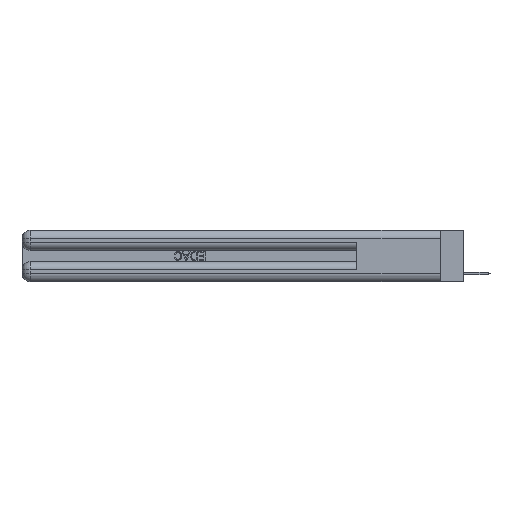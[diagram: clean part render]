
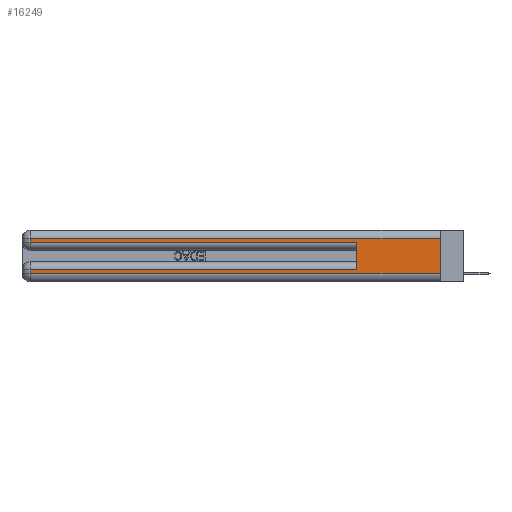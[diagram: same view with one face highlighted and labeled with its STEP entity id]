
A CAD part, left-side view. The second image highlights one B-rep face of the part: STEP entity #16249.
In plain terms, the highlighted planar face has unit normal (-1, 0, 0).
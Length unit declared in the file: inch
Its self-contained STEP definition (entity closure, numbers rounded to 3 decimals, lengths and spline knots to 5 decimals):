
#4 = ORIENTED_EDGE ( 'NONE', *, *, #17912, .T. ) ;
#371 = VERTEX_POINT ( 'NONE', #3108 ) ;
#781 = CARTESIAN_POINT ( 'NONE',  ( 0., 2.94, 0.06 ) ) ;
#1278 = CARTESIAN_POINT ( 'NONE',  ( 0., 2.94, 0.37 ) ) ;
#1391 = ORIENTED_EDGE ( 'NONE', *, *, #12706, .T. ) ;
#1417 = DIRECTION ( 'NONE',  ( 0., 0., -1. ) ) ;
#2069 = LINE ( 'NONE', #6868, #9115 ) ;
#2328 = ORIENTED_EDGE ( 'NONE', *, *, #8604, .T. ) ;
#2939 = VERTEX_POINT ( 'NONE', #16931 ) ;
#3108 = CARTESIAN_POINT ( 'NONE',  ( 0., 0.6, 0.085 ) ) ;
#4401 = EDGE_CURVE ( 'NONE', #371, #8833, #24766, .T. ) ;
#4469 = CARTESIAN_POINT ( 'NONE',  ( 0., 0., 0.06 ) ) ;
#4558 = CARTESIAN_POINT ( 'NONE',  ( 0., 0., 0.085 ) ) ;
#5405 = LINE ( 'NONE', #18814, #28959 ) ;
#5949 = CARTESIAN_POINT ( 'NONE',  ( 0., 0., 0.31 ) ) ;
#5952 = EDGE_CURVE ( 'NONE', #21578, #17408, #10750, .T. ) ;
#6176 = FACE_OUTER_BOUND ( 'NONE', #17130, .T. ) ;
#6374 = AXIS2_PLACEMENT_3D ( 'NONE', #22538, #29433, #15670 ) ;
#6868 = CARTESIAN_POINT ( 'NONE',  ( 0., 2.94, 0.37 ) ) ;
#6993 = VERTEX_POINT ( 'NONE', #17894 ) ;
#8342 = DIRECTION ( 'NONE',  ( 0., 0., 1. ) ) ;
#8559 = VECTOR ( 'NONE', #19491, 39.37008 ) ;
#8604 = EDGE_CURVE ( 'NONE', #27648, #17408, #28616, .T. ) ;
#8833 = VERTEX_POINT ( 'NONE', #12142 ) ;
#9115 = VECTOR ( 'NONE', #11151, 39.37008 ) ;
#9828 = ORIENTED_EDGE ( 'NONE', *, *, #4401, .F. ) ;
#10750 = LINE ( 'NONE', #19885, #12065 ) ;
#10819 = DIRECTION ( 'NONE',  ( 0., -1., 0. ) ) ;
#11151 = DIRECTION ( 'NONE',  ( 0., 0., -1. ) ) ;
#11373 = LINE ( 'NONE', #4558, #29319 ) ;
#11466 = VECTOR ( 'NONE', #10819, 39.37008 ) ;
#12065 = VECTOR ( 'NONE', #14960, 39.37008 ) ;
#12142 = CARTESIAN_POINT ( 'NONE',  ( 0., 0.6, 0.285 ) ) ;
#12706 = EDGE_CURVE ( 'NONE', #2939, #8833, #5405, .T. ) ;
#12940 = ORIENTED_EDGE ( 'NONE', *, *, #5952, .F. ) ;
#13879 = CARTESIAN_POINT ( 'NONE',  ( 0., 0., 0.31 ) ) ;
#14464 = DIRECTION ( 'NONE',  ( 0., -1., 0. ) ) ;
#14960 = DIRECTION ( 'NONE',  ( 0., 0., -1. ) ) ;
#15670 = DIRECTION ( 'NONE',  ( 0., 0., -1. ) ) ;
#16249 = ADVANCED_FACE ( 'NONE', ( #6176 ), #24799, .F. ) ;
#16931 = CARTESIAN_POINT ( 'NONE',  ( 0., 2.94, 0.285 ) ) ;
#17130 = EDGE_LOOP ( 'NONE', ( #12940, #20433, #24268, #1391, #9828, #4, #25158, #2328 ) ) ;
#17408 = VERTEX_POINT ( 'NONE', #4469 ) ;
#17894 = CARTESIAN_POINT ( 'NONE',  ( 0., 2.94, 0.085 ) ) ;
#17912 = EDGE_CURVE ( 'NONE', #371, #6993, #11373, .T. ) ;
#18814 = CARTESIAN_POINT ( 'NONE',  ( 0., 0., 0.285 ) ) ;
#19491 = DIRECTION ( 'NONE',  ( 0., 1., 0. ) ) ;
#19885 = CARTESIAN_POINT ( 'NONE',  ( 0., 0., 0.37 ) ) ;
#19943 = LINE ( 'NONE', #5949, #8559 ) ;
#19953 = CARTESIAN_POINT ( 'NONE',  ( 0., 2.94, 0.31 ) ) ;
#20433 = ORIENTED_EDGE ( 'NONE', *, *, #27905, .T. ) ;
#21557 = EDGE_CURVE ( 'NONE', #6993, #27648, #21728, .T. ) ;
#21578 = VERTEX_POINT ( 'NONE', #13879 ) ;
#21728 = LINE ( 'NONE', #1278, #27260 ) ;
#21902 = CARTESIAN_POINT ( 'NONE',  ( 0., 0.6, 0.145 ) ) ;
#22538 = CARTESIAN_POINT ( 'NONE',  ( 0., 0., 0.37 ) ) ;
#22578 = EDGE_CURVE ( 'NONE', #23117, #2939, #2069, .T. ) ;
#23117 = VERTEX_POINT ( 'NONE', #19953 ) ;
#24268 = ORIENTED_EDGE ( 'NONE', *, *, #22578, .T. ) ;
#24766 = LINE ( 'NONE', #21902, #27703 ) ;
#24799 = PLANE ( 'NONE',  #6374 ) ;
#25158 = ORIENTED_EDGE ( 'NONE', *, *, #21557, .T. ) ;
#26679 = CARTESIAN_POINT ( 'NONE',  ( 0., 0., 0.06 ) ) ;
#27260 = VECTOR ( 'NONE', #1417, 39.37008 ) ;
#27648 = VERTEX_POINT ( 'NONE', #781 ) ;
#27703 = VECTOR ( 'NONE', #8342, 39.37008 ) ;
#27905 = EDGE_CURVE ( 'NONE', #21578, #23117, #19943, .T. ) ;
#28616 = LINE ( 'NONE', #26679, #11466 ) ;
#28959 = VECTOR ( 'NONE', #14464, 39.37008 ) ;
#29319 = VECTOR ( 'NONE', #29477, 39.37008 ) ;
#29433 = DIRECTION ( 'NONE',  ( 1., 0., 0. ) ) ;
#29477 = DIRECTION ( 'NONE',  ( 0., 1., 0. ) ) ;
